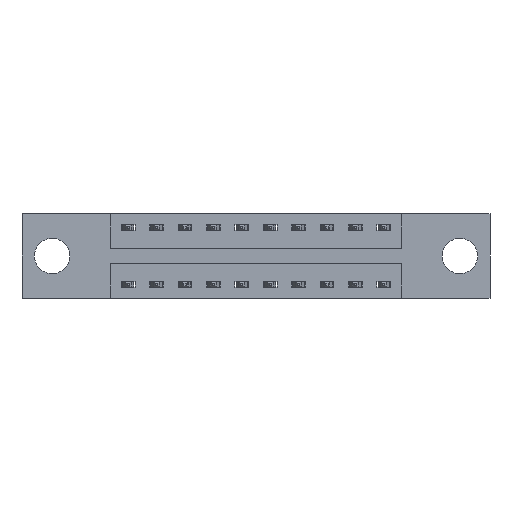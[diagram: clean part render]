
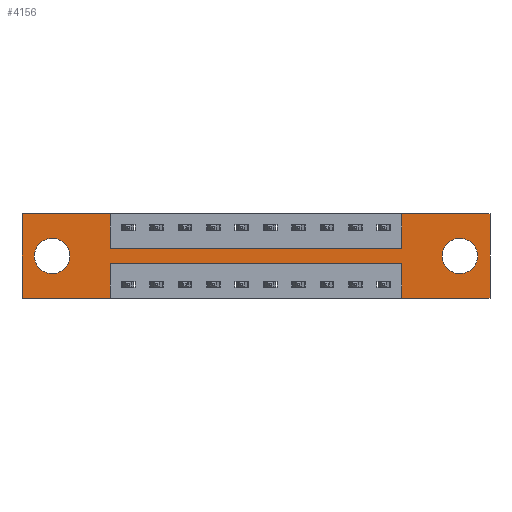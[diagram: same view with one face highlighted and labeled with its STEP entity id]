
A CAD part, front view. The second image highlights one B-rep face of the part: STEP entity #4156.
In plain terms, the highlighted planar face has unit normal (0, -1, 0).
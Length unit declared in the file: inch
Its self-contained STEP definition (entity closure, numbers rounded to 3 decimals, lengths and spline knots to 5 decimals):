
#231 = ORIENTED_EDGE ( 'NONE', *, *, #4661, .F. ) ;
#283 = DIRECTION ( 'NONE',  ( -1., 0., 0. ) ) ;
#307 = DIRECTION ( 'NONE',  ( -1., 0., 0. ) ) ;
#390 = VECTOR ( 'NONE', #4757, 39.37008 ) ;
#485 = DIRECTION ( 'NONE',  ( 0., 0., -1. ) ) ;
#551 = DIRECTION ( 'NONE',  ( -1., 0., 0. ) ) ;
#564 = VERTEX_POINT ( 'NONE', #9547 ) ;
#647 = CARTESIAN_POINT ( 'NONE',  ( 0., 0., 0. ) ) ;
#700 = DIRECTION ( 'NONE',  ( 0., 0., 1. ) ) ;
#760 = LINE ( 'NONE', #647, #7095 ) ;
#766 = LINE ( 'NONE', #4151, #5407 ) ;
#781 = VERTEX_POINT ( 'NONE', #5598 ) ;
#876 = VERTEX_POINT ( 'NONE', #2269 ) ;
#914 = DIRECTION ( 'NONE',  ( 1., 0., 0. ) ) ;
#947 = EDGE_CURVE ( 'NONE', #9203, #876, #760, .T. ) ;
#954 = LINE ( 'NONE', #10626, #7214 ) ;
#1026 = ORIENTED_EDGE ( 'NONE', *, *, #3001, .F. ) ;
#1083 = CIRCLE ( 'NONE', #2011, 0.078 ) ;
#1254 = CIRCLE ( 'NONE', #6338, 0.078 ) ;
#1276 = LINE ( 'NONE', #2263, #390 ) ;
#1587 = LINE ( 'NONE', #6860, #8420 ) ;
#1638 = DIRECTION ( 'NONE',  ( 0., 0., 1. ) ) ;
#1696 = VERTEX_POINT ( 'NONE', #4276 ) ;
#1738 = CARTESIAN_POINT ( 'NONE',  ( 0., 0., -0.37 ) ) ;
#1757 = VERTEX_POINT ( 'NONE', #5951 ) ;
#1798 = EDGE_LOOP ( 'NONE', ( #4430, #3471 ) ) ;
#1948 = LINE ( 'NONE', #9646, #5414 ) ;
#2011 = AXIS2_PLACEMENT_3D ( 'NONE', #8634, #9390, #1638 ) ;
#2016 = CARTESIAN_POINT ( 'NONE',  ( 0.3875, 0., 0. ) ) ;
#2018 = VECTOR ( 'NONE', #551, 39.37008 ) ;
#2147 = LINE ( 'NONE', #5606, #2018 ) ;
#2263 = CARTESIAN_POINT ( 'NONE',  ( 1.6725, 0., -0.37 ) ) ;
#2269 = CARTESIAN_POINT ( 'NONE',  ( 0., 0., 0. ) ) ;
#2313 = ORIENTED_EDGE ( 'NONE', *, *, #6870, .F. ) ;
#2539 = DIRECTION ( 'NONE',  ( 0., -1., 0. ) ) ;
#2572 = DIRECTION ( 'NONE',  ( 1., 0., 0. ) ) ;
#2606 = DIRECTION ( 'NONE',  ( 0., 0., -1. ) ) ;
#2667 = EDGE_LOOP ( 'NONE', ( #2313, #10470, #7390, #9239, #8162, #10807, #6298, #10828, #10541, #1026, #5262, #231 ) ) ;
#2734 = LINE ( 'NONE', #6184, #6728 ) ;
#2979 = CARTESIAN_POINT ( 'NONE',  ( 0.1325, 0., -0.263 ) ) ;
#3001 = EDGE_CURVE ( 'NONE', #876, #4464, #1587, .T. ) ;
#3206 = AXIS2_PLACEMENT_3D ( 'NONE', #6959, #8000, #11282 ) ;
#3254 = EDGE_CURVE ( 'NONE', #8799, #4719, #7021, .T. ) ;
#3471 = ORIENTED_EDGE ( 'NONE', *, *, #5161, .T. ) ;
#3573 = DIRECTION ( 'NONE',  ( 0., 0., -1. ) ) ;
#3640 = EDGE_CURVE ( 'NONE', #564, #4561, #3744, .T. ) ;
#3744 = CIRCLE ( 'NONE', #3206, 0.078 ) ;
#4012 = DIRECTION ( 'NONE',  ( 0., 1., 0. ) ) ;
#4151 = CARTESIAN_POINT ( 'NONE',  ( 0.3875, 0., -0.37 ) ) ;
#4156 = ADVANCED_FACE ( 'NONE', ( #6168, #5201, #9587 ), #8674, .T. ) ;
#4234 = CARTESIAN_POINT ( 'NONE',  ( 0.3875, 0., 0. ) ) ;
#4276 = CARTESIAN_POINT ( 'NONE',  ( 1.6725, 0., -0.22 ) ) ;
#4282 = EDGE_LOOP ( 'NONE', ( #6086, #8145 ) ) ;
#4430 = ORIENTED_EDGE ( 'NONE', *, *, #7582, .T. ) ;
#4464 = VERTEX_POINT ( 'NONE', #4234 ) ;
#4525 = LINE ( 'NONE', #8174, #9642 ) ;
#4561 = VERTEX_POINT ( 'NONE', #2979 ) ;
#4661 = EDGE_CURVE ( 'NONE', #1757, #9203, #954, .T. ) ;
#4719 = VERTEX_POINT ( 'NONE', #4959 ) ;
#4757 = DIRECTION ( 'NONE',  ( 0., 0., 1. ) ) ;
#4959 = CARTESIAN_POINT ( 'NONE',  ( 1.6725, 0., -0.15 ) ) ;
#5011 = DIRECTION ( 'NONE',  ( 0., 0., -1. ) ) ;
#5026 = VERTEX_POINT ( 'NONE', #8112 ) ;
#5161 = EDGE_CURVE ( 'NONE', #9917, #781, #9425, .T. ) ;
#5201 = FACE_BOUND ( 'NONE', #4282, .T. ) ;
#5224 = DIRECTION ( 'NONE',  ( 1., 0., 0. ) ) ;
#5262 = ORIENTED_EDGE ( 'NONE', *, *, #947, .F. ) ;
#5267 = CARTESIAN_POINT ( 'NONE',  ( 0., 0., -0.37 ) ) ;
#5407 = VECTOR ( 'NONE', #2606, 39.37008 ) ;
#5414 = VECTOR ( 'NONE', #914, 39.37008 ) ;
#5433 = VECTOR ( 'NONE', #5224, 39.37008 ) ;
#5598 = CARTESIAN_POINT ( 'NONE',  ( 1.9275, 0., -0.107 ) ) ;
#5606 = CARTESIAN_POINT ( 'NONE',  ( 0.3875, 0., -0.22 ) ) ;
#5713 = CARTESIAN_POINT ( 'NONE',  ( 1.6725, 0., 0. ) ) ;
#5799 = VERTEX_POINT ( 'NONE', #9625 ) ;
#5951 = CARTESIAN_POINT ( 'NONE',  ( 0.3875, 0., -0.37 ) ) ;
#6086 = ORIENTED_EDGE ( 'NONE', *, *, #3640, .T. ) ;
#6154 = VECTOR ( 'NONE', #7116, 39.37008 ) ;
#6168 = FACE_BOUND ( 'NONE', #1798, .T. ) ;
#6184 = CARTESIAN_POINT ( 'NONE',  ( 1.6725, 0., 0. ) ) ;
#6298 = ORIENTED_EDGE ( 'NONE', *, *, #9490, .F. ) ;
#6338 = AXIS2_PLACEMENT_3D ( 'NONE', #11125, #4012, #5011 ) ;
#6427 = VERTEX_POINT ( 'NONE', #11289 ) ;
#6558 = VERTEX_POINT ( 'NONE', #9855 ) ;
#6728 = VECTOR ( 'NONE', #7427, 39.37008 ) ;
#6860 = CARTESIAN_POINT ( 'NONE',  ( 0., 0., 0. ) ) ;
#6870 = EDGE_CURVE ( 'NONE', #5799, #1757, #766, .T. ) ;
#6938 = LINE ( 'NONE', #2016, #6154 ) ;
#6959 = CARTESIAN_POINT ( 'NONE',  ( 0.1325, 0., -0.185 ) ) ;
#7021 = LINE ( 'NONE', #10562, #5433 ) ;
#7095 = VECTOR ( 'NONE', #700, 39.37008 ) ;
#7116 = DIRECTION ( 'NONE',  ( 0., 0., -1. ) ) ;
#7165 = VERTEX_POINT ( 'NONE', #5713 ) ;
#7214 = VECTOR ( 'NONE', #283, 39.37008 ) ;
#7388 = EDGE_CURVE ( 'NONE', #4464, #8799, #6938, .T. ) ;
#7390 = ORIENTED_EDGE ( 'NONE', *, *, #10063, .F. ) ;
#7427 = DIRECTION ( 'NONE',  ( 0., 0., 1. ) ) ;
#7480 = CARTESIAN_POINT ( 'NONE',  ( 1.9275, 0., -0.263 ) ) ;
#7492 = EDGE_CURVE ( 'NONE', #7165, #6427, #1948, .T. ) ;
#7582 = EDGE_CURVE ( 'NONE', #781, #9917, #1254, .T. ) ;
#7929 = LINE ( 'NONE', #5267, #8020 ) ;
#8000 = DIRECTION ( 'NONE',  ( 0., 1., 0. ) ) ;
#8020 = VECTOR ( 'NONE', #307, 39.37008 ) ;
#8112 = CARTESIAN_POINT ( 'NONE',  ( 1.6725, 0., -0.37 ) ) ;
#8145 = ORIENTED_EDGE ( 'NONE', *, *, #9233, .T. ) ;
#8162 = ORIENTED_EDGE ( 'NONE', *, *, #8373, .F. ) ;
#8174 = CARTESIAN_POINT ( 'NONE',  ( 2.06, 0., 0. ) ) ;
#8373 = EDGE_CURVE ( 'NONE', #6427, #6558, #4525, .T. ) ;
#8420 = VECTOR ( 'NONE', #2572, 39.37008 ) ;
#8634 = CARTESIAN_POINT ( 'NONE',  ( 0.1325, 0., -0.185 ) ) ;
#8674 = PLANE ( 'NONE',  #10819 ) ;
#8799 = VERTEX_POINT ( 'NONE', #10396 ) ;
#9049 = DIRECTION ( 'NONE',  ( 0., 1., 0. ) ) ;
#9160 = CARTESIAN_POINT ( 'NONE',  ( 1.9275, 0., -0.185 ) ) ;
#9203 = VERTEX_POINT ( 'NONE', #1738 ) ;
#9233 = EDGE_CURVE ( 'NONE', #4561, #564, #1083, .T. ) ;
#9239 = ORIENTED_EDGE ( 'NONE', *, *, #9856, .F. ) ;
#9390 = DIRECTION ( 'NONE',  ( 0., 1., 0. ) ) ;
#9425 = CIRCLE ( 'NONE', #10911, 0.078 ) ;
#9490 = EDGE_CURVE ( 'NONE', #4719, #7165, #2734, .T. ) ;
#9547 = CARTESIAN_POINT ( 'NONE',  ( 0.1325, 0., -0.107 ) ) ;
#9587 = FACE_OUTER_BOUND ( 'NONE', #2667, .T. ) ;
#9589 = EDGE_CURVE ( 'NONE', #1696, #5799, #2147, .T. ) ;
#9625 = CARTESIAN_POINT ( 'NONE',  ( 0.3875, 0., -0.22 ) ) ;
#9642 = VECTOR ( 'NONE', #3573, 39.37008 ) ;
#9646 = CARTESIAN_POINT ( 'NONE',  ( 0., 0., 0. ) ) ;
#9654 = DIRECTION ( 'NONE',  ( 0., 0., -1. ) ) ;
#9855 = CARTESIAN_POINT ( 'NONE',  ( 2.06, 0., -0.37 ) ) ;
#9856 = EDGE_CURVE ( 'NONE', #6558, #5026, #7929, .T. ) ;
#9917 = VERTEX_POINT ( 'NONE', #7480 ) ;
#10063 = EDGE_CURVE ( 'NONE', #5026, #1696, #1276, .T. ) ;
#10360 = CARTESIAN_POINT ( 'NONE',  ( 0., 0., -0.37 ) ) ;
#10396 = CARTESIAN_POINT ( 'NONE',  ( 0.3875, 0., -0.15 ) ) ;
#10470 = ORIENTED_EDGE ( 'NONE', *, *, #9589, .F. ) ;
#10541 = ORIENTED_EDGE ( 'NONE', *, *, #7388, .F. ) ;
#10562 = CARTESIAN_POINT ( 'NONE',  ( 0.3875, 0., -0.15 ) ) ;
#10626 = CARTESIAN_POINT ( 'NONE',  ( 0., 0., -0.37 ) ) ;
#10807 = ORIENTED_EDGE ( 'NONE', *, *, #7492, .F. ) ;
#10819 = AXIS2_PLACEMENT_3D ( 'NONE', #10360, #2539, #9654 ) ;
#10828 = ORIENTED_EDGE ( 'NONE', *, *, #3254, .F. ) ;
#10911 = AXIS2_PLACEMENT_3D ( 'NONE', #9160, #9049, #485 ) ;
#11125 = CARTESIAN_POINT ( 'NONE',  ( 1.9275, 0., -0.185 ) ) ;
#11282 = DIRECTION ( 'NONE',  ( 0., 0., 1. ) ) ;
#11289 = CARTESIAN_POINT ( 'NONE',  ( 2.06, 0., 0. ) ) ;
